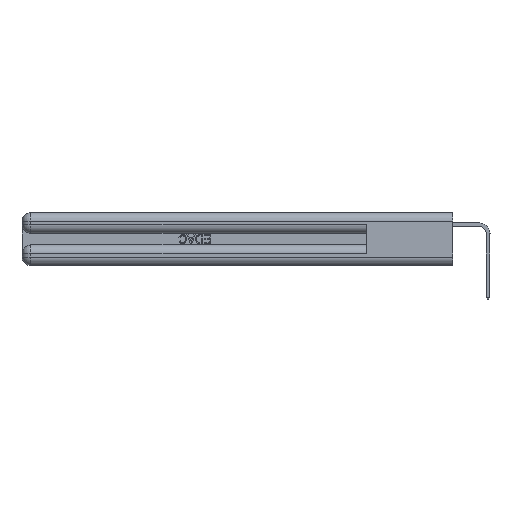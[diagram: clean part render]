
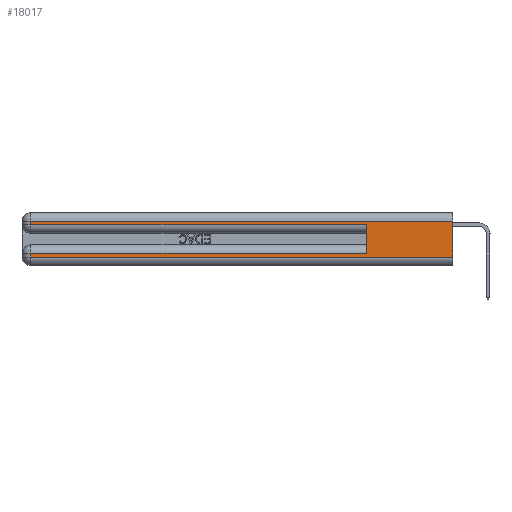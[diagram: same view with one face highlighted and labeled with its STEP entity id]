
A CAD part, left-side view. The second image highlights one B-rep face of the part: STEP entity #18017.
In plain terms, the highlighted planar face has unit normal (-1, 0, 0).
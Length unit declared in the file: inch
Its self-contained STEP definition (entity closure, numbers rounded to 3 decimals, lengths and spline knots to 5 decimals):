
#238 = ORIENTED_EDGE ( 'NONE', *, *, #20007, .T. ) ;
#2606 = CARTESIAN_POINT ( 'NONE',  ( 0., 0., 0.06 ) ) ;
#2774 = VERTEX_POINT ( 'NONE', #22988 ) ;
#3834 = PLANE ( 'NONE',  #39202 ) ;
#4198 = EDGE_CURVE ( 'NONE', #17695, #30896, #35006, .T. ) ;
#4463 = CARTESIAN_POINT ( 'NONE',  ( 0., 0.6, 0.145 ) ) ;
#4838 = DIRECTION ( 'NONE',  ( 0., 1., 0. ) ) ;
#6047 = VECTOR ( 'NONE', #36351, 39.37008 ) ;
#6150 = LINE ( 'NONE', #12471, #22133 ) ;
#6380 = EDGE_CURVE ( 'NONE', #35315, #17695, #28938, .T. ) ;
#6645 = VERTEX_POINT ( 'NONE', #36303 ) ;
#7095 = DIRECTION ( 'NONE',  ( 1., 0., 0. ) ) ;
#7339 = VERTEX_POINT ( 'NONE', #40426 ) ;
#7823 = ORIENTED_EDGE ( 'NONE', *, *, #6380, .T. ) ;
#9396 = EDGE_CURVE ( 'NONE', #7339, #6645, #6150, .T. ) ;
#9695 = CARTESIAN_POINT ( 'NONE',  ( 0., 0., 0.31 ) ) ;
#10918 = LINE ( 'NONE', #18155, #26785 ) ;
#11578 = CARTESIAN_POINT ( 'NONE',  ( 0., 0.6, 0.285 ) ) ;
#11893 = EDGE_LOOP ( 'NONE', ( #15822, #7823, #26796, #40331, #38798, #238, #29591, #14387 ) ) ;
#12078 = VECTOR ( 'NONE', #25647, 39.37008 ) ;
#12308 = DIRECTION ( 'NONE',  ( 0., -1., 0. ) ) ;
#12471 = CARTESIAN_POINT ( 'NONE',  ( 0., 2.94, 0.37 ) ) ;
#13441 = LINE ( 'NONE', #20656, #28280 ) ;
#14387 = ORIENTED_EDGE ( 'NONE', *, *, #33532, .T. ) ;
#14652 = LINE ( 'NONE', #4463, #6047 ) ;
#15170 = CARTESIAN_POINT ( 'NONE',  ( 0., 2.94, 0.31 ) ) ;
#15700 = DIRECTION ( 'NONE',  ( 0., 0., -1. ) ) ;
#15822 = ORIENTED_EDGE ( 'NONE', *, *, #16451, .F. ) ;
#16451 = EDGE_CURVE ( 'NONE', #35315, #2774, #17713, .T. ) ;
#17695 = VERTEX_POINT ( 'NONE', #15170 ) ;
#17713 = LINE ( 'NONE', #23962, #40890 ) ;
#18017 = ADVANCED_FACE ( 'NONE', ( #33870 ), #3834, .F. ) ;
#18155 = CARTESIAN_POINT ( 'NONE',  ( 0., 0., 0.285 ) ) ;
#18289 = DIRECTION ( 'NONE',  ( 0., -1., 0. ) ) ;
#20007 = EDGE_CURVE ( 'NONE', #25285, #7339, #13441, .T. ) ;
#20656 = CARTESIAN_POINT ( 'NONE',  ( 0., 0., 0.085 ) ) ;
#20971 = DIRECTION ( 'NONE',  ( 0., 0., -1. ) ) ;
#21158 = VECTOR ( 'NONE', #12308, 39.37008 ) ;
#22133 = VECTOR ( 'NONE', #15700, 39.37008 ) ;
#22988 = CARTESIAN_POINT ( 'NONE',  ( 0., 0., 0.06 ) ) ;
#23962 = CARTESIAN_POINT ( 'NONE',  ( 0., 0., 0.37 ) ) ;
#25285 = VERTEX_POINT ( 'NONE', #28492 ) ;
#25647 = DIRECTION ( 'NONE',  ( 0., 1., 0. ) ) ;
#26128 = CARTESIAN_POINT ( 'NONE',  ( 0., 0., 0.37 ) ) ;
#26332 = CARTESIAN_POINT ( 'NONE',  ( 0., 0., 0.31 ) ) ;
#26785 = VECTOR ( 'NONE', #18289, 39.37008 ) ;
#26796 = ORIENTED_EDGE ( 'NONE', *, *, #4198, .T. ) ;
#27118 = DIRECTION ( 'NONE',  ( 0., 0., -1. ) ) ;
#28280 = VECTOR ( 'NONE', #4838, 39.37008 ) ;
#28492 = CARTESIAN_POINT ( 'NONE',  ( 0., 0.6, 0.085 ) ) ;
#28938 = LINE ( 'NONE', #9695, #12078 ) ;
#29342 = DIRECTION ( 'NONE',  ( 0., 0., -1. ) ) ;
#29565 = LINE ( 'NONE', #2606, #21158 ) ;
#29591 = ORIENTED_EDGE ( 'NONE', *, *, #9396, .T. ) ;
#30896 = VERTEX_POINT ( 'NONE', #38738 ) ;
#32993 = VECTOR ( 'NONE', #20971, 39.37008 ) ;
#33532 = EDGE_CURVE ( 'NONE', #6645, #2774, #29565, .T. ) ;
#33870 = FACE_OUTER_BOUND ( 'NONE', #11893, .T. ) ;
#34878 = EDGE_CURVE ( 'NONE', #25285, #36117, #14652, .T. ) ;
#35006 = LINE ( 'NONE', #39891, #32993 ) ;
#35315 = VERTEX_POINT ( 'NONE', #26332 ) ;
#36117 = VERTEX_POINT ( 'NONE', #11578 ) ;
#36303 = CARTESIAN_POINT ( 'NONE',  ( 0., 2.94, 0.06 ) ) ;
#36351 = DIRECTION ( 'NONE',  ( 0., 0., 1. ) ) ;
#37007 = EDGE_CURVE ( 'NONE', #30896, #36117, #10918, .T. ) ;
#38738 = CARTESIAN_POINT ( 'NONE',  ( 0., 2.94, 0.285 ) ) ;
#38798 = ORIENTED_EDGE ( 'NONE', *, *, #34878, .F. ) ;
#39202 = AXIS2_PLACEMENT_3D ( 'NONE', #26128, #7095, #29342 ) ;
#39891 = CARTESIAN_POINT ( 'NONE',  ( 0., 2.94, 0.37 ) ) ;
#40331 = ORIENTED_EDGE ( 'NONE', *, *, #37007, .T. ) ;
#40426 = CARTESIAN_POINT ( 'NONE',  ( 0., 2.94, 0.085 ) ) ;
#40890 = VECTOR ( 'NONE', #27118, 39.37008 ) ;
